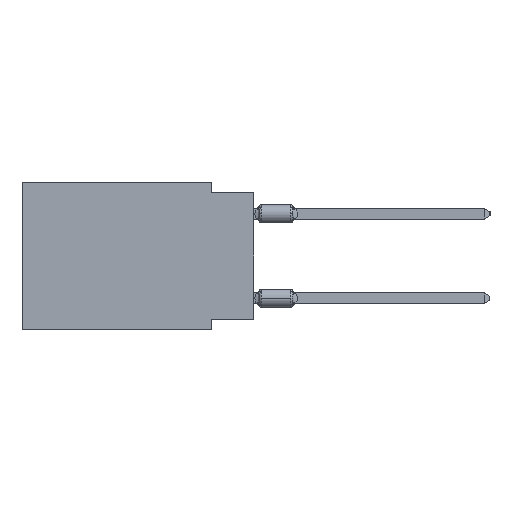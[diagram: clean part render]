
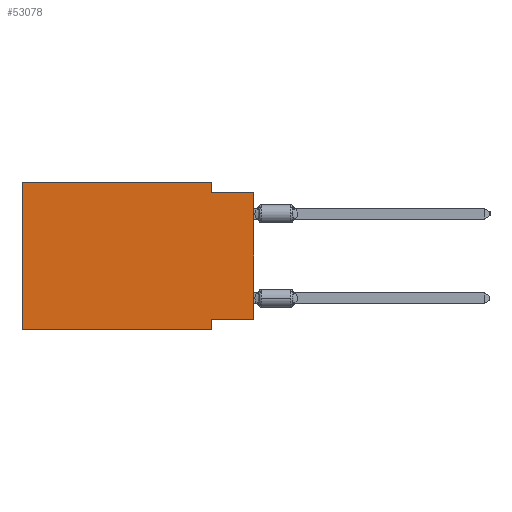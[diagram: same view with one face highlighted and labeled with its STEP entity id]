
A CAD part, left-side view. The second image highlights one B-rep face of the part: STEP entity #53078.
In plain terms, the highlighted planar face has unit normal (-1, 0, 0).
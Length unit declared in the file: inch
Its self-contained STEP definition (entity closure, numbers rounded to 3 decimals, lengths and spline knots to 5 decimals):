
#1713 = CARTESIAN_POINT ( 'NONE',  ( 0., 0.55, 0. ) ) ;
#1909 = DIRECTION ( 'NONE',  ( 0., 0., 1. ) ) ;
#2081 = EDGE_CURVE ( 'NONE', #9941, #19150, #21313, .T. ) ;
#4515 = VERTEX_POINT ( 'NONE', #4980 ) ;
#4855 = VECTOR ( 'NONE', #1909, 39.37008 ) ;
#4980 = CARTESIAN_POINT ( 'NONE',  ( 0., 0.1, 0. ) ) ;
#5067 = VECTOR ( 'NONE', #30484, 39.37008 ) ;
#5276 = DIRECTION ( 'NONE',  ( 1., 0., 0. ) ) ;
#7832 = VERTEX_POINT ( 'NONE', #62098 ) ;
#8313 = EDGE_CURVE ( 'NONE', #9941, #58506, #59783, .T. ) ;
#9941 = VERTEX_POINT ( 'NONE', #30100 ) ;
#10079 = VECTOR ( 'NONE', #43055, 39.37008 ) ;
#10667 = CARTESIAN_POINT ( 'NONE',  ( 0., 0.55, 0. ) ) ;
#10778 = FACE_OUTER_BOUND ( 'NONE', #39314, .T. ) ;
#12335 = EDGE_CURVE ( 'NONE', #4515, #33857, #53752, .T. ) ;
#13067 = CARTESIAN_POINT ( 'NONE',  ( 0., 0.55, -0.35 ) ) ;
#14255 = EDGE_CURVE ( 'NONE', #56971, #55656, #25659, .T. ) ;
#14596 = DIRECTION ( 'NONE',  ( 0., -1., 0. ) ) ;
#14703 = CARTESIAN_POINT ( 'NONE',  ( 0., 0., -0.325 ) ) ;
#17937 = VECTOR ( 'NONE', #19684, 39.37008 ) ;
#19150 = VERTEX_POINT ( 'NONE', #26506 ) ;
#19477 = EDGE_CURVE ( 'NONE', #7832, #19150, #23222, .T. ) ;
#19657 = CARTESIAN_POINT ( 'NONE',  ( 0., 0.1, 0. ) ) ;
#19684 = DIRECTION ( 'NONE',  ( 0., 1., 0. ) ) ;
#21313 = LINE ( 'NONE', #13067, #45217 ) ;
#23222 = LINE ( 'NONE', #33552, #10079 ) ;
#23654 = VECTOR ( 'NONE', #49270, 39.37008 ) ;
#25659 = LINE ( 'NONE', #41885, #62002 ) ;
#26265 = EDGE_CURVE ( 'NONE', #58506, #4515, #55241, .T. ) ;
#26506 = CARTESIAN_POINT ( 'NONE',  ( 0., 0.1, -0.35 ) ) ;
#27967 = EDGE_CURVE ( 'NONE', #56971, #7832, #42634, .T. ) ;
#28011 = DIRECTION ( 'NONE',  ( 0., -1., 0. ) ) ;
#30100 = CARTESIAN_POINT ( 'NONE',  ( 0., 0.55, -0.35 ) ) ;
#30484 = DIRECTION ( 'NONE',  ( 0., -1., 0. ) ) ;
#30559 = ORIENTED_EDGE ( 'NONE', *, *, #2081, .T. ) ;
#30941 = CARTESIAN_POINT ( 'NONE',  ( 0., 0.1, -0.025 ) ) ;
#33552 = CARTESIAN_POINT ( 'NONE',  ( 0., 0.1, -0.35 ) ) ;
#33721 = ORIENTED_EDGE ( 'NONE', *, *, #14255, .T. ) ;
#33857 = VERTEX_POINT ( 'NONE', #30941 ) ;
#39314 = EDGE_LOOP ( 'NONE', ( #33721, #53864, #51713, #59144, #39611, #30559, #62469, #59422 ) ) ;
#39611 = ORIENTED_EDGE ( 'NONE', *, *, #8313, .F. ) ;
#39638 = DIRECTION ( 'NONE',  ( 0., 0., -1. ) ) ;
#39887 = CARTESIAN_POINT ( 'NONE',  ( 0., 0.55, 0. ) ) ;
#41885 = CARTESIAN_POINT ( 'NONE',  ( 0., 0., 0. ) ) ;
#42634 = LINE ( 'NONE', #14703, #17937 ) ;
#43055 = DIRECTION ( 'NONE',  ( 0., 0., -1. ) ) ;
#45212 = PLANE ( 'NONE',  #57827 ) ;
#45217 = VECTOR ( 'NONE', #28011, 39.37008 ) ;
#46224 = CARTESIAN_POINT ( 'NONE',  ( 0., 0.55, 0. ) ) ;
#46906 = CARTESIAN_POINT ( 'NONE',  ( 0., 0., -0.325 ) ) ;
#49270 = DIRECTION ( 'NONE',  ( 0., 0., -1. ) ) ;
#51713 = ORIENTED_EDGE ( 'NONE', *, *, #12335, .F. ) ;
#53078 = ADVANCED_FACE ( 'NONE', ( #10778 ), #45212, .F. ) ;
#53684 = VECTOR ( 'NONE', #14596, 39.37008 ) ;
#53752 = LINE ( 'NONE', #19657, #23654 ) ;
#53766 = LINE ( 'NONE', #54457, #5067 ) ;
#53864 = ORIENTED_EDGE ( 'NONE', *, *, #63640, .F. ) ;
#54457 = CARTESIAN_POINT ( 'NONE',  ( 0., 0., -0.025 ) ) ;
#55241 = LINE ( 'NONE', #39887, #53684 ) ;
#55656 = VERTEX_POINT ( 'NONE', #58057 ) ;
#56971 = VERTEX_POINT ( 'NONE', #46906 ) ;
#57827 = AXIS2_PLACEMENT_3D ( 'NONE', #10667, #5276, #39638 ) ;
#58057 = CARTESIAN_POINT ( 'NONE',  ( 0., 0., -0.025 ) ) ;
#58506 = VERTEX_POINT ( 'NONE', #1713 ) ;
#59144 = ORIENTED_EDGE ( 'NONE', *, *, #26265, .F. ) ;
#59422 = ORIENTED_EDGE ( 'NONE', *, *, #27967, .F. ) ;
#59783 = LINE ( 'NONE', #46224, #4855 ) ;
#60779 = DIRECTION ( 'NONE',  ( 0., 0., 1. ) ) ;
#62002 = VECTOR ( 'NONE', #60779, 39.37008 ) ;
#62098 = CARTESIAN_POINT ( 'NONE',  ( 0., 0.1, -0.325 ) ) ;
#62469 = ORIENTED_EDGE ( 'NONE', *, *, #19477, .F. ) ;
#63640 = EDGE_CURVE ( 'NONE', #33857, #55656, #53766, .T. ) ;
